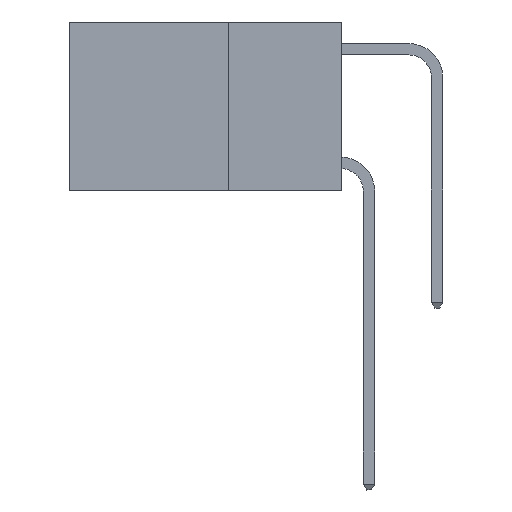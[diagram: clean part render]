
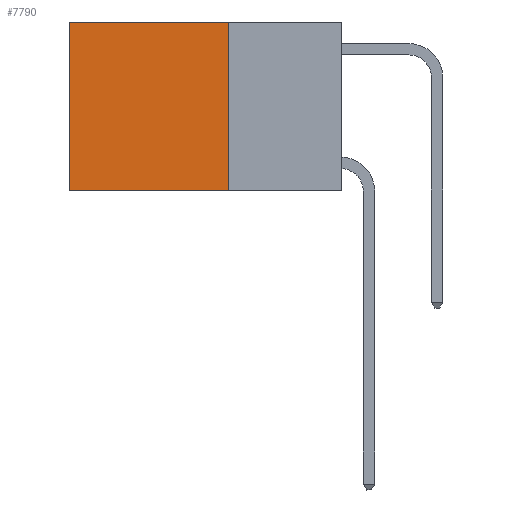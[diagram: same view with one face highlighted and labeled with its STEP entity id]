
A CAD part, left-side view. The second image highlights one B-rep face of the part: STEP entity #7790.
In plain terms, the highlighted planar face has unit normal (-1, 0, 0).
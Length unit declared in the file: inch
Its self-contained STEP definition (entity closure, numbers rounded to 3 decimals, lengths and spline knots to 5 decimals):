
#195 = EDGE_LOOP ( 'NONE', ( #5507, #12133, #12218, #4510 ) ) ;
#1651 = EDGE_CURVE ( 'NONE', #10483, #6370, #8801, .T. ) ;
#1921 = AXIS2_PLACEMENT_3D ( 'NONE', #9361, #14330, #7842 ) ;
#2139 = LINE ( 'NONE', #12066, #4589 ) ;
#2159 = VERTEX_POINT ( 'NONE', #7199 ) ;
#2180 = LINE ( 'NONE', #15864, #7205 ) ;
#3612 = VECTOR ( 'NONE', #12044, 39.37008 ) ;
#3899 = VECTOR ( 'NONE', #16188, 39.37008 ) ;
#4510 = ORIENTED_EDGE ( 'NONE', *, *, #8030, .T. ) ;
#4589 = VECTOR ( 'NONE', #13438, 39.37008 ) ;
#5507 = ORIENTED_EDGE ( 'NONE', *, *, #14407, .T. ) ;
#6370 = VERTEX_POINT ( 'NONE', #7748 ) ;
#6487 = CARTESIAN_POINT ( 'NONE',  ( 0.2625, 0.25, -0.37 ) ) ;
#6845 = FACE_OUTER_BOUND ( 'NONE', #195, .T. ) ;
#7199 = CARTESIAN_POINT ( 'NONE',  ( 0.2625, 0.6, 0. ) ) ;
#7205 = VECTOR ( 'NONE', #12180, 39.37008 ) ;
#7748 = CARTESIAN_POINT ( 'NONE',  ( 0.2625, 0.6, -0.37 ) ) ;
#7790 = ADVANCED_FACE ( 'NONE', ( #6845 ), #14082, .F. ) ;
#7842 = DIRECTION ( 'NONE',  ( 0., 0., -1. ) ) ;
#8030 = EDGE_CURVE ( 'NONE', #15686, #2159, #2180, .T. ) ;
#8801 = LINE ( 'NONE', #14932, #3899 ) ;
#9361 = CARTESIAN_POINT ( 'NONE',  ( 0.2625, 0.25, 0. ) ) ;
#10362 = CARTESIAN_POINT ( 'NONE',  ( 0.2625, 0.25, 0. ) ) ;
#10483 = VERTEX_POINT ( 'NONE', #6487 ) ;
#10721 = LINE ( 'NONE', #11957, #3612 ) ;
#11932 = EDGE_CURVE ( 'NONE', #15686, #10483, #10721, .T. ) ;
#11957 = CARTESIAN_POINT ( 'NONE',  ( 0.2625, 0.25, 0. ) ) ;
#12044 = DIRECTION ( 'NONE',  ( 0., 0., -1. ) ) ;
#12066 = CARTESIAN_POINT ( 'NONE',  ( 0.2625, 0.6, 0. ) ) ;
#12133 = ORIENTED_EDGE ( 'NONE', *, *, #1651, .F. ) ;
#12180 = DIRECTION ( 'NONE',  ( 0., 1., 0. ) ) ;
#12218 = ORIENTED_EDGE ( 'NONE', *, *, #11932, .F. ) ;
#13438 = DIRECTION ( 'NONE',  ( 0., 0., -1. ) ) ;
#14082 = PLANE ( 'NONE',  #1921 ) ;
#14330 = DIRECTION ( 'NONE',  ( 1., 0., 0. ) ) ;
#14407 = EDGE_CURVE ( 'NONE', #2159, #6370, #2139, .T. ) ;
#14932 = CARTESIAN_POINT ( 'NONE',  ( 0.2625, 0.25, -0.37 ) ) ;
#15686 = VERTEX_POINT ( 'NONE', #10362 ) ;
#15864 = CARTESIAN_POINT ( 'NONE',  ( 0.2625, 0.25, 0. ) ) ;
#16188 = DIRECTION ( 'NONE',  ( 0., 1., 0. ) ) ;
